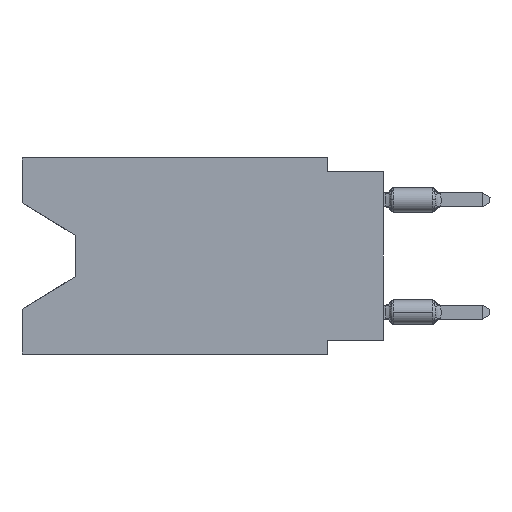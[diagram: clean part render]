
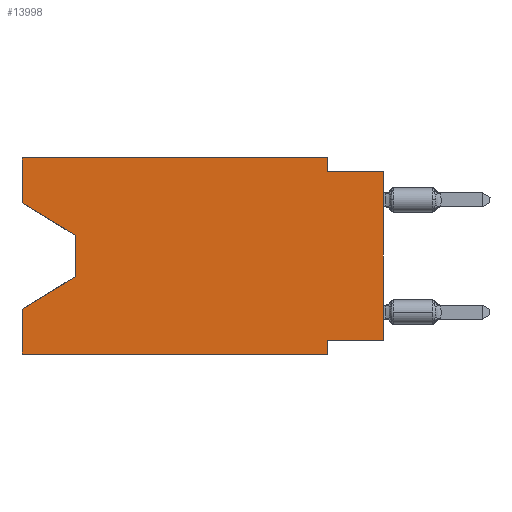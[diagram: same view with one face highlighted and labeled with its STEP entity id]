
A CAD part, left-side view. The second image highlights one B-rep face of the part: STEP entity #13998.
In plain terms, the highlighted planar face has unit normal (-1, 0, 0).
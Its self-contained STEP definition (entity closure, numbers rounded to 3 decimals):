
#92 = CARTESIAN_POINT ( 'NONE',  ( 0., 13.97, -3.505 ) ) ;
#506 = CARTESIAN_POINT ( 'NONE',  ( 0., 0., -0.635 ) ) ;
#1263 = DIRECTION ( 'NONE',  ( 0., 0., -1. ) ) ;
#1299 = FACE_OUTER_BOUND ( 'NONE', #7442, .T. ) ;
#1360 = CARTESIAN_POINT ( 'NONE',  ( 0., 2.54, -8.89 ) ) ;
#1426 = CARTESIAN_POINT ( 'NONE',  ( 0., 13.97, -5.385 ) ) ;
#1628 = EDGE_CURVE ( 'NONE', #20065, #3675, #21405, .T. ) ;
#2266 = CARTESIAN_POINT ( 'NONE',  ( 0., 0., -8.255 ) ) ;
#2450 = VECTOR ( 'NONE', #35680, 1000. ) ;
#2591 = VECTOR ( 'NONE', #5127, 1000. ) ;
#2651 = EDGE_CURVE ( 'NONE', #28130, #9216, #16703, .T. ) ;
#3675 = VERTEX_POINT ( 'NONE', #7817 ) ;
#4271 = PLANE ( 'NONE',  #34339 ) ;
#4427 = EDGE_CURVE ( 'NONE', #14566, #9216, #34487, .T. ) ;
#4586 = VERTEX_POINT ( 'NONE', #21495 ) ;
#4593 = CARTESIAN_POINT ( 'NONE',  ( 0., 16.383, -8.89 ) ) ;
#4971 = CARTESIAN_POINT ( 'NONE',  ( 0., 16.383, 0. ) ) ;
#5127 = DIRECTION ( 'NONE',  ( 0., 0., -1. ) ) ;
#5217 = ORIENTED_EDGE ( 'NONE', *, *, #18320, .T. ) ;
#5534 = DIRECTION ( 'NONE',  ( 0., 0., 1. ) ) ;
#5670 = LINE ( 'NONE', #92, #2591 ) ;
#5716 = LINE ( 'NONE', #36723, #13346 ) ;
#6188 = DIRECTION ( 'NONE',  ( 0., -1., 0. ) ) ;
#6898 = CARTESIAN_POINT ( 'NONE',  ( 0., 16.383, -2.038 ) ) ;
#7442 = EDGE_LOOP ( 'NONE', ( #35801, #23716, #5217, #18045, #36204, #18344, #20966, #30283, #14816, #17481, #7494, #11890 ) ) ;
#7494 = ORIENTED_EDGE ( 'NONE', *, *, #7614, .F. ) ;
#7612 = VERTEX_POINT ( 'NONE', #1360 ) ;
#7614 = EDGE_CURVE ( 'NONE', #8692, #30427, #20874, .T. ) ;
#7817 = CARTESIAN_POINT ( 'NONE',  ( 0., 13.97, -3.505 ) ) ;
#8544 = DIRECTION ( 'NONE',  ( 0., 0., -1. ) ) ;
#8692 = VERTEX_POINT ( 'NONE', #4971 ) ;
#9035 = EDGE_CURVE ( 'NONE', #28130, #4586, #35890, .T. ) ;
#9216 = VERTEX_POINT ( 'NONE', #26405 ) ;
#10062 = CARTESIAN_POINT ( 'NONE',  ( 0., 13.97, -5.385 ) ) ;
#10398 = DIRECTION ( 'NONE',  ( 1., 0., 0. ) ) ;
#10523 = LINE ( 'NONE', #1426, #36655 ) ;
#10840 = DIRECTION ( 'NONE',  ( 0., 0., 1. ) ) ;
#10932 = DIRECTION ( 'NONE',  ( 0., 0., -1. ) ) ;
#11389 = CARTESIAN_POINT ( 'NONE',  ( 0., 16.383, -2.038 ) ) ;
#11890 = ORIENTED_EDGE ( 'NONE', *, *, #27696, .F. ) ;
#12530 = CARTESIAN_POINT ( 'NONE',  ( 0., 16.383, -6.852 ) ) ;
#12822 = EDGE_CURVE ( 'NONE', #4586, #7612, #32842, .T. ) ;
#13346 = VECTOR ( 'NONE', #5534, 1000. ) ;
#13943 = CARTESIAN_POINT ( 'NONE',  ( 0., 2.54, 0. ) ) ;
#13998 = ADVANCED_FACE ( 'NONE', ( #1299 ), #4271, .F. ) ;
#14566 = VERTEX_POINT ( 'NONE', #35559 ) ;
#14816 = ORIENTED_EDGE ( 'NONE', *, *, #4427, .F. ) ;
#14983 = DIRECTION ( 'NONE',  ( 0., -1., 0. ) ) ;
#15600 = CARTESIAN_POINT ( 'NONE',  ( 0., 16.383, 0. ) ) ;
#16703 = LINE ( 'NONE', #19689, #27436 ) ;
#16845 = VECTOR ( 'NONE', #10840, 1000. ) ;
#16906 = LINE ( 'NONE', #13943, #31141 ) ;
#17481 = ORIENTED_EDGE ( 'NONE', *, *, #25412, .F. ) ;
#18045 = ORIENTED_EDGE ( 'NONE', *, *, #36135, .F. ) ;
#18277 = CARTESIAN_POINT ( 'NONE',  ( 0., 16.383, 0. ) ) ;
#18320 = EDGE_CURVE ( 'NONE', #34538, #26304, #10523, .T. ) ;
#18344 = ORIENTED_EDGE ( 'NONE', *, *, #12822, .F. ) ;
#19689 = CARTESIAN_POINT ( 'NONE',  ( 0., 0., 0. ) ) ;
#20065 = VERTEX_POINT ( 'NONE', #11389 ) ;
#20874 = LINE ( 'NONE', #18277, #32384 ) ;
#20966 = ORIENTED_EDGE ( 'NONE', *, *, #9035, .F. ) ;
#21331 = LINE ( 'NONE', #4593, #36370 ) ;
#21405 = LINE ( 'NONE', #6898, #2450 ) ;
#21495 = CARTESIAN_POINT ( 'NONE',  ( 0., 2.54, -8.255 ) ) ;
#21799 = CARTESIAN_POINT ( 'NONE',  ( 0., 0., -8.255 ) ) ;
#22586 = VERTEX_POINT ( 'NONE', #35447 ) ;
#23716 = ORIENTED_EDGE ( 'NONE', *, *, #27229, .T. ) ;
#24461 = DIRECTION ( 'NONE',  ( 0., 0.855, -0.519 ) ) ;
#24649 = DIRECTION ( 'NONE',  ( 0., -1., 0. ) ) ;
#25412 = EDGE_CURVE ( 'NONE', #30427, #14566, #16906, .T. ) ;
#26304 = VERTEX_POINT ( 'NONE', #12530 ) ;
#26405 = CARTESIAN_POINT ( 'NONE',  ( 0., 0., -0.635 ) ) ;
#27229 = EDGE_CURVE ( 'NONE', #3675, #34538, #5670, .T. ) ;
#27394 = CARTESIAN_POINT ( 'NONE',  ( 0., 16.383, 0. ) ) ;
#27436 = VECTOR ( 'NONE', #28045, 1000. ) ;
#27696 = EDGE_CURVE ( 'NONE', #20065, #8692, #30351, .T. ) ;
#28045 = DIRECTION ( 'NONE',  ( 0., 0., 1. ) ) ;
#28130 = VERTEX_POINT ( 'NONE', #2266 ) ;
#28916 = VECTOR ( 'NONE', #30507, 1000. ) ;
#30283 = ORIENTED_EDGE ( 'NONE', *, *, #2651, .T. ) ;
#30351 = LINE ( 'NONE', #27394, #16845 ) ;
#30427 = VERTEX_POINT ( 'NONE', #34166 ) ;
#30507 = DIRECTION ( 'NONE',  ( 0., 1., 0. ) ) ;
#31141 = VECTOR ( 'NONE', #8544, 1000. ) ;
#32384 = VECTOR ( 'NONE', #6188, 1000. ) ;
#32842 = LINE ( 'NONE', #35622, #34373 ) ;
#34166 = CARTESIAN_POINT ( 'NONE',  ( 0., 2.54, 0. ) ) ;
#34339 = AXIS2_PLACEMENT_3D ( 'NONE', #15600, #10398, #10932 ) ;
#34373 = VECTOR ( 'NONE', #1263, 1000. ) ;
#34487 = LINE ( 'NONE', #506, #35708 ) ;
#34538 = VERTEX_POINT ( 'NONE', #10062 ) ;
#35447 = CARTESIAN_POINT ( 'NONE',  ( 0., 16.383, -8.89 ) ) ;
#35559 = CARTESIAN_POINT ( 'NONE',  ( 0., 2.54, -0.635 ) ) ;
#35622 = CARTESIAN_POINT ( 'NONE',  ( 0., 2.54, -8.89 ) ) ;
#35680 = DIRECTION ( 'NONE',  ( 0., -0.855, -0.519 ) ) ;
#35708 = VECTOR ( 'NONE', #14983, 1000. ) ;
#35801 = ORIENTED_EDGE ( 'NONE', *, *, #1628, .T. ) ;
#35890 = LINE ( 'NONE', #21799, #28916 ) ;
#36135 = EDGE_CURVE ( 'NONE', #22586, #26304, #5716, .T. ) ;
#36204 = ORIENTED_EDGE ( 'NONE', *, *, #36504, .T. ) ;
#36370 = VECTOR ( 'NONE', #24649, 1000. ) ;
#36504 = EDGE_CURVE ( 'NONE', #22586, #7612, #21331, .T. ) ;
#36655 = VECTOR ( 'NONE', #24461, 1000. ) ;
#36723 = CARTESIAN_POINT ( 'NONE',  ( 0., 16.383, 0. ) ) ;
